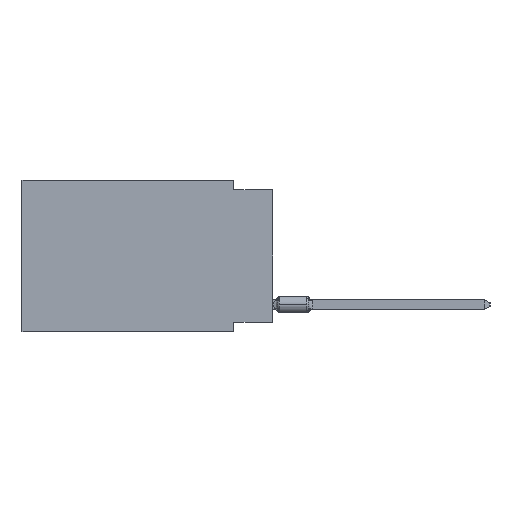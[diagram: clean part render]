
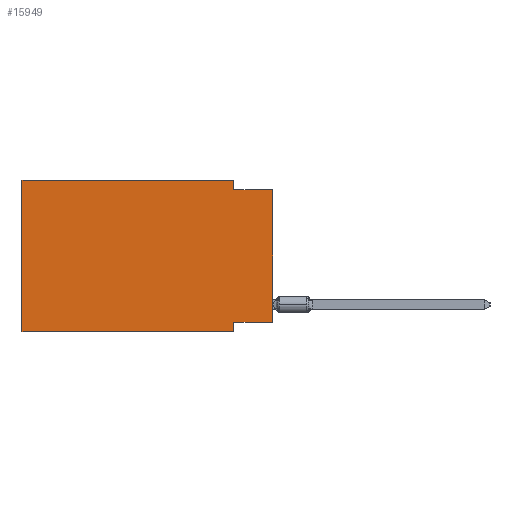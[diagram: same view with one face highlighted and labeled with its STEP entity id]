
A CAD part, left-side view. The second image highlights one B-rep face of the part: STEP entity #15949.
In plain terms, the highlighted planar face has unit normal (-1, 0, 0).
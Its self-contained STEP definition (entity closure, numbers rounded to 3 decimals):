
#986 = VERTEX_POINT ( 'NONE', #24116 ) ;
#1787 = CARTESIAN_POINT ( 'NONE',  ( 0., 16.383, -9.906 ) ) ;
#2958 = EDGE_LOOP ( 'NONE', ( #42008, #39173, #8956, #47581, #48808, #37499, #56159, #40970 ) ) ;
#4257 = CARTESIAN_POINT ( 'NONE',  ( 0., 0., 0. ) ) ;
#4960 = VERTEX_POINT ( 'NONE', #46227 ) ;
#7752 = DIRECTION ( 'NONE',  ( 0., 0., -1. ) ) ;
#8375 = CARTESIAN_POINT ( 'NONE',  ( 0., 16.383, 0. ) ) ;
#8377 = CARTESIAN_POINT ( 'NONE',  ( 0., 2.54, -9.906 ) ) ;
#8956 = ORIENTED_EDGE ( 'NONE', *, *, #29483, .F. ) ;
#10028 = VECTOR ( 'NONE', #39457, 1000. ) ;
#10965 = VERTEX_POINT ( 'NONE', #8377 ) ;
#11430 = CARTESIAN_POINT ( 'NONE',  ( 0., 0., -0.635 ) ) ;
#12349 = LINE ( 'NONE', #11430, #31748 ) ;
#12972 = LINE ( 'NONE', #41238, #36176 ) ;
#15949 = ADVANCED_FACE ( 'NONE', ( #51395 ), #55786, .F. ) ;
#16414 = CARTESIAN_POINT ( 'NONE',  ( 0., 2.54, 0. ) ) ;
#20606 = LINE ( 'NONE', #1787, #10028 ) ;
#21074 = AXIS2_PLACEMENT_3D ( 'NONE', #8375, #41965, #46368 ) ;
#23679 = DIRECTION ( 'NONE',  ( 0., 0., 1. ) ) ;
#24116 = CARTESIAN_POINT ( 'NONE',  ( 0., 2.54, -9.271 ) ) ;
#24314 = VECTOR ( 'NONE', #46429, 1000. ) ;
#26551 = VECTOR ( 'NONE', #7752, 1000. ) ;
#29483 = EDGE_CURVE ( 'NONE', #43221, #4960, #59565, .T. ) ;
#30764 = VECTOR ( 'NONE', #23679, 1000. ) ;
#31748 = VECTOR ( 'NONE', #60082, 1000. ) ;
#32498 = LINE ( 'NONE', #4257, #30764 ) ;
#32711 = VERTEX_POINT ( 'NONE', #38937 ) ;
#35895 = DIRECTION ( 'NONE',  ( 0., 0., -1. ) ) ;
#36176 = VECTOR ( 'NONE', #35895, 1000. ) ;
#36503 = VERTEX_POINT ( 'NONE', #51625 ) ;
#37499 = ORIENTED_EDGE ( 'NONE', *, *, #57529, .T. ) ;
#38937 = CARTESIAN_POINT ( 'NONE',  ( 0., 0., -0.635 ) ) ;
#39073 = EDGE_CURVE ( 'NONE', #56385, #36503, #55781, .T. ) ;
#39173 = ORIENTED_EDGE ( 'NONE', *, *, #53612, .F. ) ;
#39457 = DIRECTION ( 'NONE',  ( 0., -1., 0. ) ) ;
#40970 = ORIENTED_EDGE ( 'NONE', *, *, #58503, .F. ) ;
#41238 = CARTESIAN_POINT ( 'NONE',  ( 0., 2.54, -9.906 ) ) ;
#41965 = DIRECTION ( 'NONE',  ( 1., 0., 0. ) ) ;
#42008 = ORIENTED_EDGE ( 'NONE', *, *, #53389, .T. ) ;
#43221 = VERTEX_POINT ( 'NONE', #16414 ) ;
#44976 = LINE ( 'NONE', #54696, #24314 ) ;
#45492 = VECTOR ( 'NONE', #46064, 1000. ) ;
#45749 = CARTESIAN_POINT ( 'NONE',  ( 0., 16.383, 0. ) ) ;
#46064 = DIRECTION ( 'NONE',  ( 0., 0., 1. ) ) ;
#46198 = VECTOR ( 'NONE', #60014, 1000. ) ;
#46227 = CARTESIAN_POINT ( 'NONE',  ( 0., 2.54, -0.635 ) ) ;
#46368 = DIRECTION ( 'NONE',  ( 0., 0., -1. ) ) ;
#46429 = DIRECTION ( 'NONE',  ( 0., -1., 0. ) ) ;
#47581 = ORIENTED_EDGE ( 'NONE', *, *, #60770, .F. ) ;
#48808 = ORIENTED_EDGE ( 'NONE', *, *, #39073, .F. ) ;
#49529 = CARTESIAN_POINT ( 'NONE',  ( 0., 0., -9.271 ) ) ;
#50804 = VERTEX_POINT ( 'NONE', #49529 ) ;
#50892 = CARTESIAN_POINT ( 'NONE',  ( 0., 0., -9.271 ) ) ;
#51395 = FACE_OUTER_BOUND ( 'NONE', #2958, .T. ) ;
#51625 = CARTESIAN_POINT ( 'NONE',  ( 0., 16.383, 0. ) ) ;
#51889 = CARTESIAN_POINT ( 'NONE',  ( 0., 16.383, -9.906 ) ) ;
#53389 = EDGE_CURVE ( 'NONE', #50804, #32711, #32498, .T. ) ;
#53612 = EDGE_CURVE ( 'NONE', #4960, #32711, #12349, .T. ) ;
#54696 = CARTESIAN_POINT ( 'NONE',  ( 0., 16.383, 0. ) ) ;
#55781 = LINE ( 'NONE', #45749, #45492 ) ;
#55786 = PLANE ( 'NONE',  #21074 ) ;
#56159 = ORIENTED_EDGE ( 'NONE', *, *, #58158, .F. ) ;
#56385 = VERTEX_POINT ( 'NONE', #51889 ) ;
#57529 = EDGE_CURVE ( 'NONE', #56385, #10965, #20606, .T. ) ;
#58158 = EDGE_CURVE ( 'NONE', #986, #10965, #12972, .T. ) ;
#58503 = EDGE_CURVE ( 'NONE', #50804, #986, #60320, .T. ) ;
#59257 = CARTESIAN_POINT ( 'NONE',  ( 0., 2.54, 0. ) ) ;
#59565 = LINE ( 'NONE', #59257, #26551 ) ;
#60014 = DIRECTION ( 'NONE',  ( 0., 1., 0. ) ) ;
#60082 = DIRECTION ( 'NONE',  ( 0., -1., 0. ) ) ;
#60320 = LINE ( 'NONE', #50892, #46198 ) ;
#60770 = EDGE_CURVE ( 'NONE', #36503, #43221, #44976, .T. ) ;
